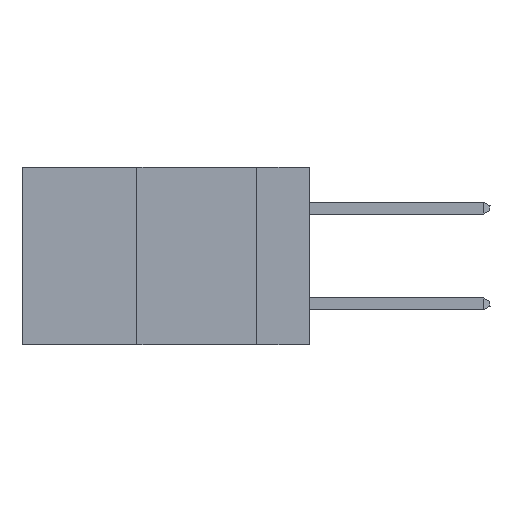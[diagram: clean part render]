
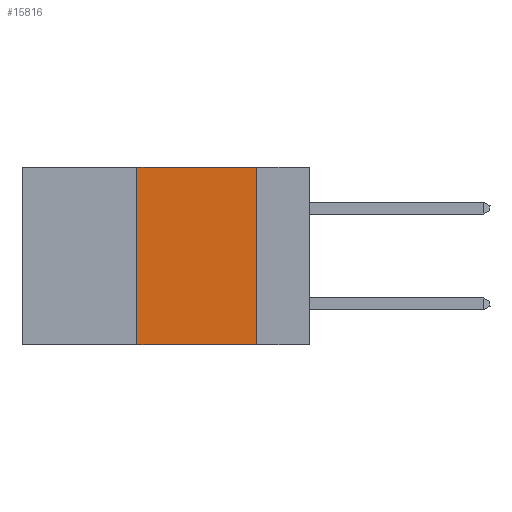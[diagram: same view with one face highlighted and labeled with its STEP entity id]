
A CAD part, left-side view. The second image highlights one B-rep face of the part: STEP entity #15816.
In plain terms, the highlighted planar face has unit normal (-1, 0, 0).
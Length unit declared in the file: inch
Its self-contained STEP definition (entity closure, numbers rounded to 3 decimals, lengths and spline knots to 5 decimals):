
#243 = FACE_OUTER_BOUND ( 'NONE', #34452, .T. ) ;
#2125 = PLANE ( 'NONE',  #27763 ) ;
#6180 = VECTOR ( 'NONE', #21087, 39.37008 ) ;
#6207 = EDGE_CURVE ( 'NONE', #7827, #26400, #25378, .T. ) ;
#7076 = ORIENTED_EDGE ( 'NONE', *, *, #35697, .F. ) ;
#7827 = VERTEX_POINT ( 'NONE', #14002 ) ;
#12494 = DIRECTION ( 'NONE',  ( 1., 0., 0. ) ) ;
#12968 = ORIENTED_EDGE ( 'NONE', *, *, #45482, .T. ) ;
#13745 = DIRECTION ( 'NONE',  ( 0., 0., -1. ) ) ;
#14002 = CARTESIAN_POINT ( 'NONE',  ( 0., 0.36, 0. ) ) ;
#14501 = VERTEX_POINT ( 'NONE', #40846 ) ;
#14556 = LINE ( 'NONE', #32012, #31315 ) ;
#14692 = CARTESIAN_POINT ( 'NONE',  ( 0., 0.6, -0.37 ) ) ;
#15816 = ADVANCED_FACE ( 'NONE', ( #243 ), #2125, .F. ) ;
#17424 = ORIENTED_EDGE ( 'NONE', *, *, #6207, .F. ) ;
#18535 = CARTESIAN_POINT ( 'NONE',  ( 0., 0.36, 0. ) ) ;
#21087 = DIRECTION ( 'NONE',  ( 0., -1., 0. ) ) ;
#22132 = VERTEX_POINT ( 'NONE', #33319 ) ;
#23280 = DIRECTION ( 'NONE',  ( 0., 0., -1. ) ) ;
#25135 = LINE ( 'NONE', #14692, #6180 ) ;
#25378 = LINE ( 'NONE', #28949, #44251 ) ;
#25845 = LINE ( 'NONE', #18535, #38652 ) ;
#26400 = VERTEX_POINT ( 'NONE', #36504 ) ;
#27763 = AXIS2_PLACEMENT_3D ( 'NONE', #30469, #12494, #23280 ) ;
#28949 = CARTESIAN_POINT ( 'NONE',  ( 0., 0.6, 0. ) ) ;
#30469 = CARTESIAN_POINT ( 'NONE',  ( 0., 0.6, 0. ) ) ;
#31315 = VECTOR ( 'NONE', #13745, 39.37008 ) ;
#32012 = CARTESIAN_POINT ( 'NONE',  ( 0., 0.11, 0. ) ) ;
#33319 = CARTESIAN_POINT ( 'NONE',  ( 0., 0.36, -0.37 ) ) ;
#34452 = EDGE_LOOP ( 'NONE', ( #7076, #17424, #45464, #12968 ) ) ;
#35656 = DIRECTION ( 'NONE',  ( 0., 0., 1. ) ) ;
#35697 = EDGE_CURVE ( 'NONE', #26400, #14501, #14556, .T. ) ;
#36504 = CARTESIAN_POINT ( 'NONE',  ( 0., 0.11, 0. ) ) ;
#38479 = EDGE_CURVE ( 'NONE', #22132, #7827, #25845, .T. ) ;
#38652 = VECTOR ( 'NONE', #35656, 39.37008 ) ;
#39824 = DIRECTION ( 'NONE',  ( 0., -1., 0. ) ) ;
#40846 = CARTESIAN_POINT ( 'NONE',  ( 0., 0.11, -0.37 ) ) ;
#44251 = VECTOR ( 'NONE', #39824, 39.37008 ) ;
#45464 = ORIENTED_EDGE ( 'NONE', *, *, #38479, .F. ) ;
#45482 = EDGE_CURVE ( 'NONE', #22132, #14501, #25135, .T. ) ;
